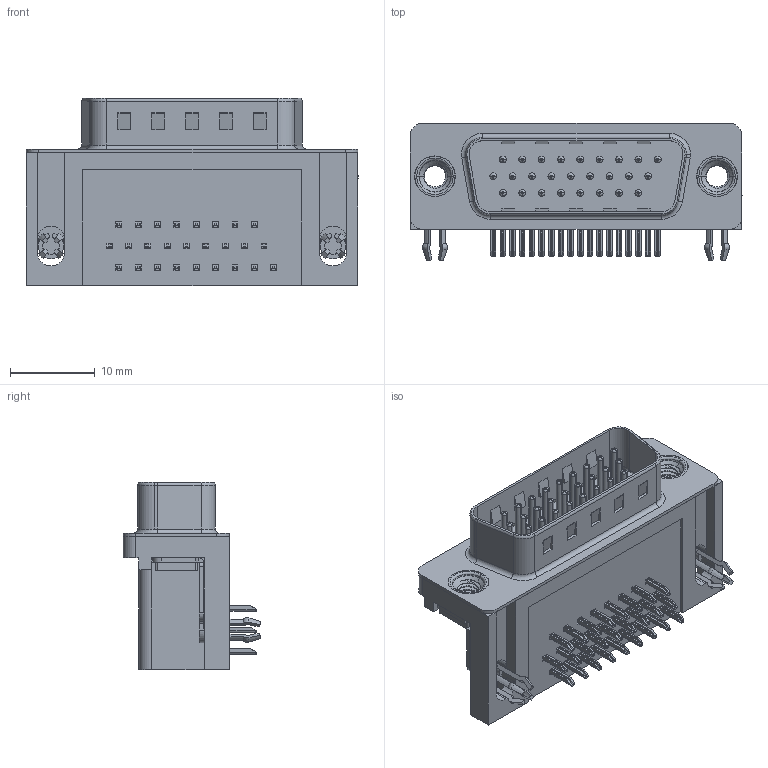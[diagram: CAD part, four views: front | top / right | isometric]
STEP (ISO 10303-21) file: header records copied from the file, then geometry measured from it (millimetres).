
FILE_DESCRIPTION (( 'STEP AP203' ), '1' );
FILE_NAME ('633-026-263-545.STEP', '2018-11-09T00:03:56', ( '' ), ( '' ), 'SwSTEP 2.0', 'SolidWorks 2016', '' );
FILE_SCHEMA (( 'CONFIG_CONTROL_DESIGN' ));
Length unit declared in the file: millimetre
Products named in the file (8): 633 Housing_26 Contact; 633 Shell_26 Contact; 633 Contact Bottom; 633 Contact Middle; 633 Contact Top; 633 4 Prong Board Lock; 633 M3 Threaded Rivet; 633-026-263-545
Assembly tree (32 placements, depth 2):
  633-026-263-545
    633 Housing_26 Contact
    633 Shell_26 Contact
    633 Contact Bottom  x8
    633 Contact Middle  x9
    633 Contact Top  x9
    633 4 Prong Board Lock  x2
    633 M3 Threaded Rivet  x2
Bounding box: 39.22 x 16.25 x 22.1 mm (x, y, z)
Volume: 5602.1 mm3; surface area: 7327.5 mm2
Topology: 32 solids, 32 shells, 2424 faces, 6056 edges, 3755 vertices
Faces by surface type: plane 1463, cylinder 688, torus 219, cone 48, bspline 6
Entity records: 25524 total; most frequent: CARTESIAN_POINT 5370, DIRECTION 3999, ORIENTED_EDGE 3800, EDGE_CURVE 1900, AXIS2_PLACEMENT_3D 1364, VECTOR 1271, LINE 1271, VERTEX_POINT 1218
